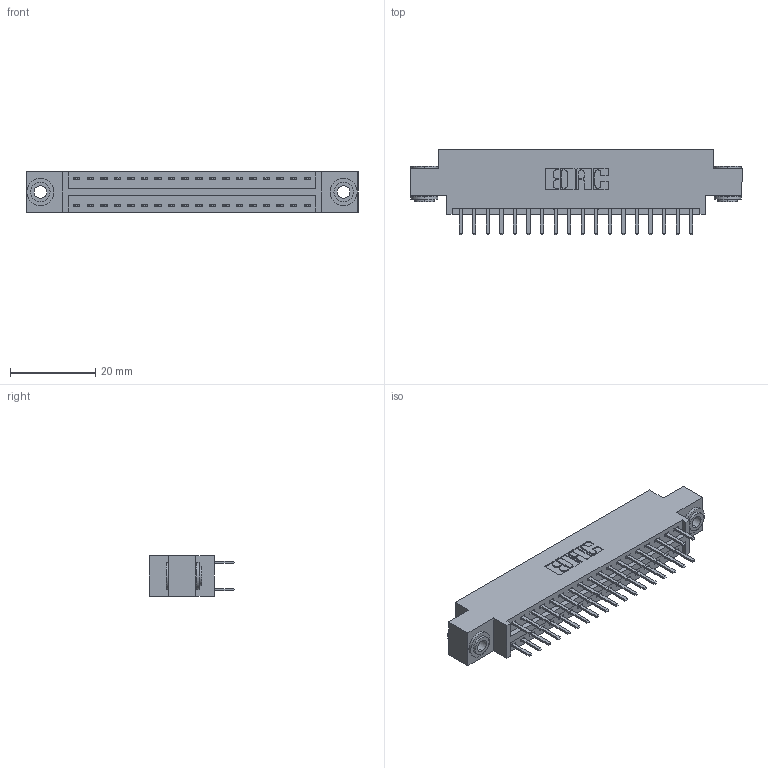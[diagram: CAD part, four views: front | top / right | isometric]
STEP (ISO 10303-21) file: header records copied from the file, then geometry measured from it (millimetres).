
FILE_DESCRIPTION (( 'STEP AP203' ), '1' );
FILE_NAME ('346-036-520-803.STEP', '2022-05-19T21:00:42', ( '' ), ( '' ), 'SwSTEP 2.0', 'SolidWorks 2020', '' );
FILE_SCHEMA (( 'CONFIG_CONTROL_DESIGN' ));
Length unit declared in the file: inch
Products named in the file (4): 345-292-001_345-293-120; 346 Part_0.170 Offset - 0.156 Dia-TH; 345-250-002_345-250-002-102; 346-036-520-803
Assembly tree (39 placements, depth 2):
  346-036-520-803
    346 Part_0.170 Offset - 0.156 Dia-TH
    345-292-001_345-293-120  x36
    345-250-002_345-250-002-102  x2
Bounding box: 77.72 x 20.02 x 9.4 mm (x, y, z)
Volume: 7223.5 mm3; surface area: 9943.2 mm2
Topology: 39 solids, 39 shells, 2194 faces, 6321 edges, 4114 vertices
Faces by surface type: plane 1436, cylinder 750, cone 8
Entity records: 16290 total; most frequent: CARTESIAN_POINT 2713, ORIENTED_EDGE 2626, DIRECTION 2459, EDGE_CURVE 1313, VECTOR 1081, LINE 1081, VERTEX_POINT 870, AXIS2_PLACEMENT_3D 689
